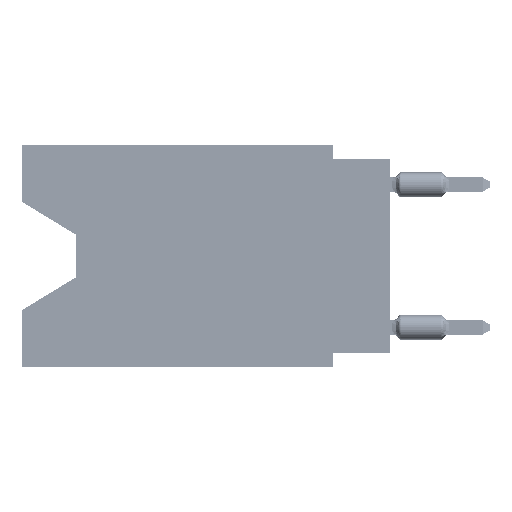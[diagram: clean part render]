
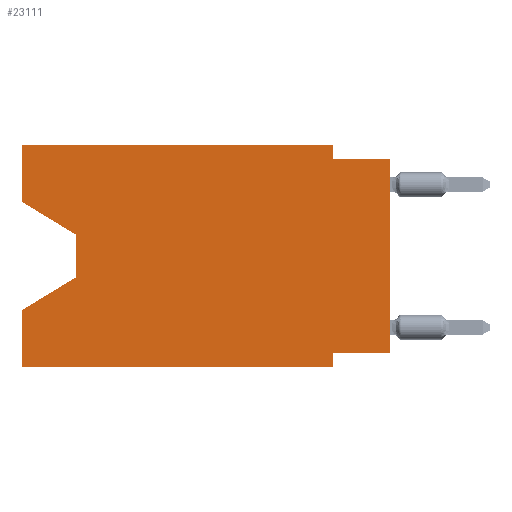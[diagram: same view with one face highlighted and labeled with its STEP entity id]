
A CAD part, left-side view. The second image highlights one B-rep face of the part: STEP entity #23111.
In plain terms, the highlighted planar face has unit normal (-1, 0, 0).
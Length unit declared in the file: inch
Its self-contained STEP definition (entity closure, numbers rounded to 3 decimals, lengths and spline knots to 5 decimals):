
#255 = DIRECTION ( 'NONE',  ( 0., 0., 1. ) ) ;
#2616 = ORIENTED_EDGE ( 'NONE', *, *, #12933, .T. ) ;
#4161 = CARTESIAN_POINT ( 'NONE',  ( 0., 0., 0. ) ) ;
#5232 = LINE ( 'NONE', #44897, #79362 ) ;
#5521 = CARTESIAN_POINT ( 'NONE',  ( 0., 0.55, -0.232 ) ) ;
#6439 = VERTEX_POINT ( 'NONE', #64209 ) ;
#7997 = CARTESIAN_POINT ( 'NONE',  ( 0., 0.645, 0. ) ) ;
#8608 = CARTESIAN_POINT ( 'NONE',  ( 0., 0.1, -0.365 ) ) ;
#10506 = CARTESIAN_POINT ( 'NONE',  ( 0., 0.645, -0.39 ) ) ;
#11439 = FACE_OUTER_BOUND ( 'NONE', #38371, .T. ) ;
#11595 = ORIENTED_EDGE ( 'NONE', *, *, #14074, .F. ) ;
#11748 = DIRECTION ( 'NONE',  ( 0., -1., 0. ) ) ;
#12933 = EDGE_CURVE ( 'NONE', #60627, #21532, #15178, .T. ) ;
#13364 = VECTOR ( 'NONE', #53791, 39.37008 ) ;
#13505 = CARTESIAN_POINT ( 'NONE',  ( 0., 0., -0.365 ) ) ;
#14074 = EDGE_CURVE ( 'NONE', #23878, #37340, #48144, .T. ) ;
#15178 = LINE ( 'NONE', #29764, #58269 ) ;
#16108 = VECTOR ( 'NONE', #25649, 39.37008 ) ;
#16974 = DIRECTION ( 'NONE',  ( 0., 0., 1. ) ) ;
#17046 = CARTESIAN_POINT ( 'NONE',  ( 0., 0.1, 0. ) ) ;
#17448 = CARTESIAN_POINT ( 'NONE',  ( 0., 0.55, -0.158 ) ) ;
#17725 = CARTESIAN_POINT ( 'NONE',  ( 0., 0.645, 0. ) ) ;
#18715 = LINE ( 'NONE', #66572, #13364 ) ;
#19086 = DIRECTION ( 'NONE',  ( 0., -1., 0. ) ) ;
#19731 = CARTESIAN_POINT ( 'NONE',  ( 0., 0.645, -0.28975 ) ) ;
#20646 = CARTESIAN_POINT ( 'NONE',  ( 0., 0., -0.025 ) ) ;
#21158 = VERTEX_POINT ( 'NONE', #75424 ) ;
#21532 = VERTEX_POINT ( 'NONE', #19731 ) ;
#21942 = EDGE_CURVE ( 'NONE', #37340, #72453, #18715, .T. ) ;
#22037 = VECTOR ( 'NONE', #27182, 39.37008 ) ;
#23111 = ADVANCED_FACE ( 'NONE', ( #11439 ), #73890, .F. ) ;
#23815 = LINE ( 'NONE', #51614, #48095 ) ;
#23878 = VERTEX_POINT ( 'NONE', #68785 ) ;
#23890 = DIRECTION ( 'NONE',  ( 0., 0., -1. ) ) ;
#25649 = DIRECTION ( 'NONE',  ( 0., 0., -1. ) ) ;
#25699 = LINE ( 'NONE', #17046, #77177 ) ;
#27182 = DIRECTION ( 'NONE',  ( 0., 1., 0. ) ) ;
#29764 = CARTESIAN_POINT ( 'NONE',  ( 0., 0.55, -0.232 ) ) ;
#29825 = EDGE_CURVE ( 'NONE', #23878, #63673, #33747, .T. ) ;
#32053 = LINE ( 'NONE', #17448, #16108 ) ;
#33747 = LINE ( 'NONE', #4161, #34486 ) ;
#34486 = VECTOR ( 'NONE', #61082, 39.37008 ) ;
#36139 = DIRECTION ( 'NONE',  ( 0., 0.855, -0.519 ) ) ;
#37340 = VERTEX_POINT ( 'NONE', #8608 ) ;
#38371 = EDGE_LOOP ( 'NONE', ( #55071, #42010, #2616, #61790, #45493, #89485, #11595, #63035, #45961, #66684, #66845, #46902 ) ) ;
#40991 = VERTEX_POINT ( 'NONE', #81802 ) ;
#41230 = EDGE_CURVE ( 'NONE', #68415, #60627, #32053, .T. ) ;
#41514 = LINE ( 'NONE', #61098, #50354 ) ;
#42010 = ORIENTED_EDGE ( 'NONE', *, *, #41230, .T. ) ;
#44203 = VERTEX_POINT ( 'NONE', #56887 ) ;
#44897 = CARTESIAN_POINT ( 'NONE',  ( 0., 0.645, -0.10025 ) ) ;
#45493 = ORIENTED_EDGE ( 'NONE', *, *, #45604, .T. ) ;
#45604 = EDGE_CURVE ( 'NONE', #77593, #72453, #53226, .T. ) ;
#45961 = ORIENTED_EDGE ( 'NONE', *, *, #87164, .F. ) ;
#46902 = ORIENTED_EDGE ( 'NONE', *, *, #47375, .F. ) ;
#46935 = AXIS2_PLACEMENT_3D ( 'NONE', #53808, #74795, #75659 ) ;
#47375 = EDGE_CURVE ( 'NONE', #21158, #6439, #55397, .T. ) ;
#48095 = VECTOR ( 'NONE', #16974, 39.37008 ) ;
#48144 = LINE ( 'NONE', #13505, #22037 ) ;
#48309 = DIRECTION ( 'NONE',  ( 0., -1., 0. ) ) ;
#50354 = VECTOR ( 'NONE', #48309, 39.37008 ) ;
#51614 = CARTESIAN_POINT ( 'NONE',  ( 0., 0.645, 0. ) ) ;
#53226 = LINE ( 'NONE', #81030, #73373 ) ;
#53791 = DIRECTION ( 'NONE',  ( 0., 0., -1. ) ) ;
#53808 = CARTESIAN_POINT ( 'NONE',  ( 0., 0.645, 0. ) ) ;
#55071 = ORIENTED_EDGE ( 'NONE', *, *, #65304, .T. ) ;
#55397 = LINE ( 'NONE', #7997, #66064 ) ;
#56887 = CARTESIAN_POINT ( 'NONE',  ( 0., 0.1, 0. ) ) ;
#58269 = VECTOR ( 'NONE', #36139, 39.37008 ) ;
#60627 = VERTEX_POINT ( 'NONE', #5521 ) ;
#61082 = DIRECTION ( 'NONE',  ( 0., 0., 1. ) ) ;
#61098 = CARTESIAN_POINT ( 'NONE',  ( 0., 0., -0.025 ) ) ;
#61749 = CARTESIAN_POINT ( 'NONE',  ( 0., 0.1, -0.39 ) ) ;
#61790 = ORIENTED_EDGE ( 'NONE', *, *, #75902, .F. ) ;
#63035 = ORIENTED_EDGE ( 'NONE', *, *, #29825, .T. ) ;
#63673 = VERTEX_POINT ( 'NONE', #20646 ) ;
#63679 = VECTOR ( 'NONE', #19086, 39.37008 ) ;
#64209 = CARTESIAN_POINT ( 'NONE',  ( 0., 0.645, 0. ) ) ;
#65304 = EDGE_CURVE ( 'NONE', #21158, #68415, #5232, .T. ) ;
#66064 = VECTOR ( 'NONE', #255, 39.37008 ) ;
#66572 = CARTESIAN_POINT ( 'NONE',  ( 0., 0.1, -0.39 ) ) ;
#66684 = ORIENTED_EDGE ( 'NONE', *, *, #74035, .F. ) ;
#66845 = ORIENTED_EDGE ( 'NONE', *, *, #88706, .F. ) ;
#67210 = DIRECTION ( 'NONE',  ( 0., -0.855, -0.519 ) ) ;
#67394 = LINE ( 'NONE', #17725, #63679 ) ;
#68415 = VERTEX_POINT ( 'NONE', #88632 ) ;
#68785 = CARTESIAN_POINT ( 'NONE',  ( 0., 0., -0.365 ) ) ;
#72453 = VERTEX_POINT ( 'NONE', #61749 ) ;
#73373 = VECTOR ( 'NONE', #11748, 39.37008 ) ;
#73890 = PLANE ( 'NONE',  #46935 ) ;
#74035 = EDGE_CURVE ( 'NONE', #44203, #40991, #25699, .T. ) ;
#74795 = DIRECTION ( 'NONE',  ( 1., 0., 0. ) ) ;
#75424 = CARTESIAN_POINT ( 'NONE',  ( 0., 0.645, -0.10025 ) ) ;
#75659 = DIRECTION ( 'NONE',  ( 0., 0., -1. ) ) ;
#75902 = EDGE_CURVE ( 'NONE', #77593, #21532, #23815, .T. ) ;
#77177 = VECTOR ( 'NONE', #23890, 39.37008 ) ;
#77593 = VERTEX_POINT ( 'NONE', #10506 ) ;
#79362 = VECTOR ( 'NONE', #67210, 39.37008 ) ;
#81030 = CARTESIAN_POINT ( 'NONE',  ( 0., 0.645, -0.39 ) ) ;
#81802 = CARTESIAN_POINT ( 'NONE',  ( 0., 0.1, -0.025 ) ) ;
#87164 = EDGE_CURVE ( 'NONE', #40991, #63673, #41514, .T. ) ;
#88632 = CARTESIAN_POINT ( 'NONE',  ( 0., 0.55, -0.158 ) ) ;
#88706 = EDGE_CURVE ( 'NONE', #6439, #44203, #67394, .T. ) ;
#89485 = ORIENTED_EDGE ( 'NONE', *, *, #21942, .F. ) ;
